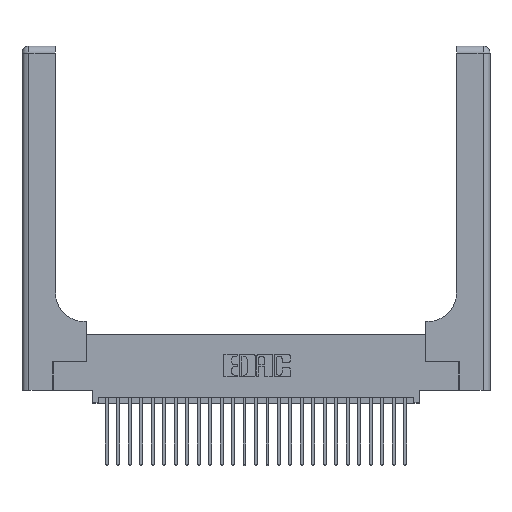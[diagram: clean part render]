
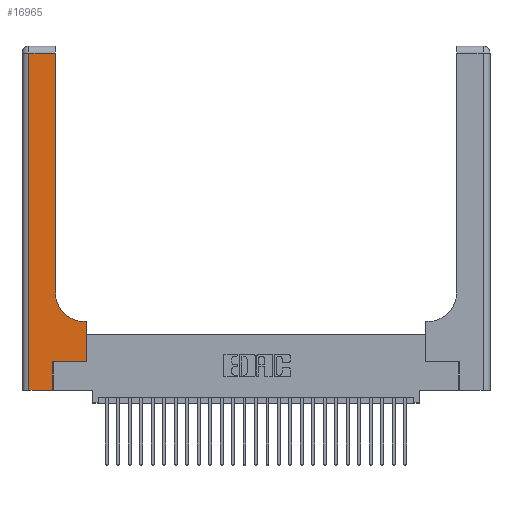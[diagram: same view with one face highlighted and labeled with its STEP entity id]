
A CAD part, top view. The second image highlights one B-rep face of the part: STEP entity #16965.
In plain terms, the highlighted planar face has unit normal (0, 0, 1).
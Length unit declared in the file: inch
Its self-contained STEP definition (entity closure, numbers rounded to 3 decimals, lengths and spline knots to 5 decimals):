
#260 = CARTESIAN_POINT ( 'NONE',  ( 0.5415, 0.6, 0.37 ) ) ;
#351 = ORIENTED_EDGE ( 'NONE', *, *, #19321, .T. ) ;
#1013 = DIRECTION ( 'NONE',  ( 0., 1., 0. ) ) ;
#1157 = ORIENTED_EDGE ( 'NONE', *, *, #15932, .T. ) ;
#1217 = VERTEX_POINT ( 'NONE', #16977 ) ;
#1426 = VECTOR ( 'NONE', #23952, 39.37008 ) ;
#1533 = AXIS2_PLACEMENT_3D ( 'NONE', #16719, #21145, #12379 ) ;
#2492 = VECTOR ( 'NONE', #13536, 39.37008 ) ;
#2615 = EDGE_CURVE ( 'NONE', #11067, #1217, #24911, .T. ) ;
#3760 = DIRECTION ( 'NONE',  ( -1., 0., 0. ) ) ;
#4538 = ORIENTED_EDGE ( 'NONE', *, *, #8038, .T. ) ;
#4588 = ORIENTED_EDGE ( 'NONE', *, *, #5280, .T. ) ;
#5280 = EDGE_CURVE ( 'NONE', #16141, #28054, #15791, .T. ) ;
#6046 = VECTOR ( 'NONE', #14054, 39.37008 ) ;
#6053 = DIRECTION ( 'NONE',  ( 1., 0., 0. ) ) ;
#6350 = CARTESIAN_POINT ( 'NONE',  ( 0.269, 0., 0.37 ) ) ;
#6941 = CARTESIAN_POINT ( 'NONE',  ( 0.5415, 0.85, 0.37 ) ) ;
#7375 = CARTESIAN_POINT ( 'NONE',  ( 0.06, 0., 0.37 ) ) ;
#8038 = EDGE_CURVE ( 'NONE', #16100, #12825, #8685, .T. ) ;
#8685 = LINE ( 'NONE', #23268, #2492 ) ;
#8883 = VECTOR ( 'NONE', #6053, 39.37008 ) ;
#10640 = FACE_OUTER_BOUND ( 'NONE', #26706, .T. ) ;
#10671 = ORIENTED_EDGE ( 'NONE', *, *, #12809, .T. ) ;
#10979 = LINE ( 'NONE', #14218, #25461 ) ;
#11067 = VERTEX_POINT ( 'NONE', #16814 ) ;
#11476 = VERTEX_POINT ( 'NONE', #24232 ) ;
#12379 = DIRECTION ( 'NONE',  ( -1., 0., 0. ) ) ;
#12809 = EDGE_CURVE ( 'NONE', #1217, #16141, #13652, .T. ) ;
#12825 = VERTEX_POINT ( 'NONE', #7375 ) ;
#13194 = CARTESIAN_POINT ( 'NONE',  ( 0.06, 2.94, 0.37 ) ) ;
#13349 = CARTESIAN_POINT ( 'NONE',  ( 0.5585, 0.25, 0.37 ) ) ;
#13536 = DIRECTION ( 'NONE',  ( 0., -1., 0. ) ) ;
#13652 = LINE ( 'NONE', #20707, #6046 ) ;
#13670 = VECTOR ( 'NONE', #21188, 39.37008 ) ;
#13716 = DIRECTION ( 'NONE',  ( 1., 0., 0. ) ) ;
#14054 = DIRECTION ( 'NONE',  ( -1., 0., 0. ) ) ;
#14218 = CARTESIAN_POINT ( 'NONE',  ( 0.269, 0., 0.37 ) ) ;
#14503 = VECTOR ( 'NONE', #3760, 39.37008 ) ;
#14654 = AXIS2_PLACEMENT_3D ( 'NONE', #6941, #26906, #13716 ) ;
#14749 = CARTESIAN_POINT ( 'NONE',  ( 0., 0., 0.37 ) ) ;
#14967 = CARTESIAN_POINT ( 'NONE',  ( 0., 2.94, 0.37 ) ) ;
#15209 = LINE ( 'NONE', #14967, #14503 ) ;
#15791 = CIRCLE ( 'NONE', #14654, 0.25 ) ;
#15932 = EDGE_CURVE ( 'NONE', #11476, #16100, #15209, .T. ) ;
#16100 = VERTEX_POINT ( 'NONE', #13194 ) ;
#16141 = VERTEX_POINT ( 'NONE', #260 ) ;
#16719 = CARTESIAN_POINT ( 'NONE',  ( 0., 3., 0.37 ) ) ;
#16814 = CARTESIAN_POINT ( 'NONE',  ( 0.5585, 0.25, 0.37 ) ) ;
#16850 = LINE ( 'NONE', #14749, #8883 ) ;
#16965 = ADVANCED_FACE ( 'NONE', ( #10640 ), #25267, .F. ) ;
#16977 = CARTESIAN_POINT ( 'NONE',  ( 0.5585, 0.6, 0.37 ) ) ;
#17046 = EDGE_CURVE ( 'NONE', #12825, #25173, #16850, .T. ) ;
#17226 = VERTEX_POINT ( 'NONE', #24791 ) ;
#18464 = ORIENTED_EDGE ( 'NONE', *, *, #23948, .T. ) ;
#19321 = EDGE_CURVE ( 'NONE', #28054, #11476, #27092, .T. ) ;
#20707 = CARTESIAN_POINT ( 'NONE',  ( 0.2915, 0.6, 0.37 ) ) ;
#21145 = DIRECTION ( 'NONE',  ( 0., 0., -1. ) ) ;
#21188 = DIRECTION ( 'NONE',  ( 0., 1., 0. ) ) ;
#21458 = VECTOR ( 'NONE', #26224, 39.37008 ) ;
#21467 = CARTESIAN_POINT ( 'NONE',  ( 0.269, 0.25, 0.37 ) ) ;
#21695 = ORIENTED_EDGE ( 'NONE', *, *, #28537, .T. ) ;
#22116 = LINE ( 'NONE', #21467, #1426 ) ;
#22253 = CARTESIAN_POINT ( 'NONE',  ( 0.2915, 0.85, 0.37 ) ) ;
#23060 = ORIENTED_EDGE ( 'NONE', *, *, #2615, .T. ) ;
#23268 = CARTESIAN_POINT ( 'NONE',  ( 0.06, 3., 0.37 ) ) ;
#23787 = ORIENTED_EDGE ( 'NONE', *, *, #17046, .T. ) ;
#23948 = EDGE_CURVE ( 'NONE', #17226, #11067, #22116, .T. ) ;
#23952 = DIRECTION ( 'NONE',  ( 1., 0., 0. ) ) ;
#24232 = CARTESIAN_POINT ( 'NONE',  ( 0.2915, 2.94, 0.37 ) ) ;
#24791 = CARTESIAN_POINT ( 'NONE',  ( 0.269, 0.25, 0.37 ) ) ;
#24911 = LINE ( 'NONE', #13349, #21458 ) ;
#25173 = VERTEX_POINT ( 'NONE', #6350 ) ;
#25267 = PLANE ( 'NONE',  #1533 ) ;
#25461 = VECTOR ( 'NONE', #1013, 39.37008 ) ;
#26224 = DIRECTION ( 'NONE',  ( 0., 1., 0. ) ) ;
#26706 = EDGE_LOOP ( 'NONE', ( #351, #1157, #4538, #23787, #21695, #18464, #23060, #10671, #4588 ) ) ;
#26906 = DIRECTION ( 'NONE',  ( 0., 0., -1. ) ) ;
#27092 = LINE ( 'NONE', #27718, #13670 ) ;
#27718 = CARTESIAN_POINT ( 'NONE',  ( 0.2915, 3., 0.37 ) ) ;
#28054 = VERTEX_POINT ( 'NONE', #22253 ) ;
#28537 = EDGE_CURVE ( 'NONE', #25173, #17226, #10979, .T. ) ;
